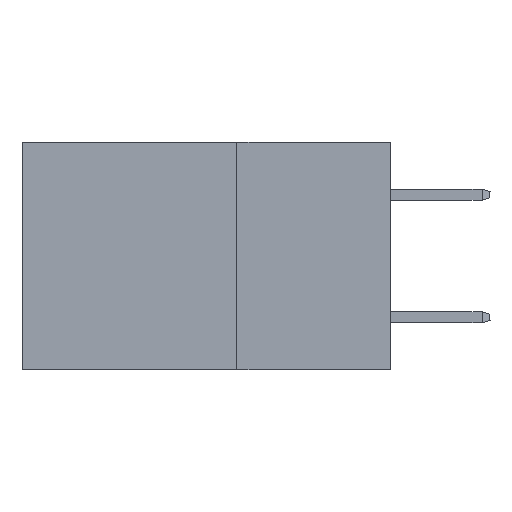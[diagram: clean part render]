
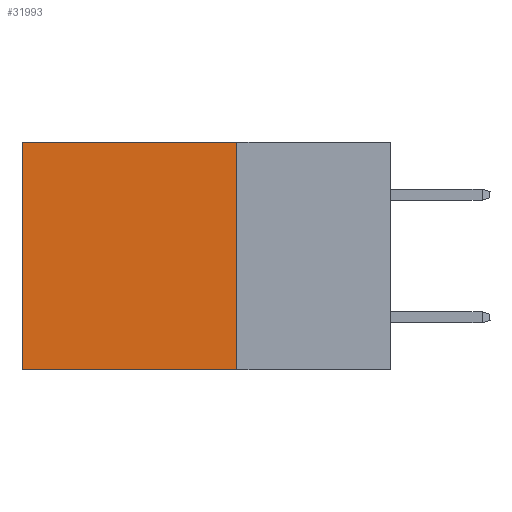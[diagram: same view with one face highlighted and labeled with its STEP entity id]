
A CAD part, left-side view. The second image highlights one B-rep face of the part: STEP entity #31993.
In plain terms, the highlighted planar face has unit normal (-1, 0, 0).
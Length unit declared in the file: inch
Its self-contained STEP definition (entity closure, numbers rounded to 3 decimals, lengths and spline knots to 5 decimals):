
#470 = VECTOR ( 'NONE', #37193, 39.37008 ) ;
#1246 = VECTOR ( 'NONE', #6303, 39.37008 ) ;
#2619 = AXIS2_PLACEMENT_3D ( 'NONE', #25971, #29019, #23151 ) ;
#3380 = VERTEX_POINT ( 'NONE', #5142 ) ;
#3623 = LINE ( 'NONE', #7963, #470 ) ;
#5142 = CARTESIAN_POINT ( 'NONE',  ( 0.2875, 0.25, 0. ) ) ;
#5642 = ORIENTED_EDGE ( 'NONE', *, *, #17626, .F. ) ;
#5778 = VECTOR ( 'NONE', #6934, 39.37008 ) ;
#5882 = CARTESIAN_POINT ( 'NONE',  ( 0.2875, 0.25, -0.37 ) ) ;
#6303 = DIRECTION ( 'NONE',  ( 0., 0., -1. ) ) ;
#6636 = ORIENTED_EDGE ( 'NONE', *, *, #25671, .T. ) ;
#6934 = DIRECTION ( 'NONE',  ( 0., 0., -1. ) ) ;
#7260 = VERTEX_POINT ( 'NONE', #5882 ) ;
#7963 = CARTESIAN_POINT ( 'NONE',  ( 0.2875, 0.25, 0. ) ) ;
#8611 = ORIENTED_EDGE ( 'NONE', *, *, #31252, .T. ) ;
#8920 = LINE ( 'NONE', #23599, #1246 ) ;
#10044 = CARTESIAN_POINT ( 'NONE',  ( 0.2875, 0.25, -0.37 ) ) ;
#10802 = VERTEX_POINT ( 'NONE', #28279 ) ;
#12981 = DIRECTION ( 'NONE',  ( 0., 1., 0. ) ) ;
#13115 = FACE_OUTER_BOUND ( 'NONE', #36855, .T. ) ;
#16904 = CARTESIAN_POINT ( 'NONE',  ( 0.2875, 0.6, 0. ) ) ;
#17626 = EDGE_CURVE ( 'NONE', #7260, #10802, #22421, .T. ) ;
#20752 = ORIENTED_EDGE ( 'NONE', *, *, #25717, .F. ) ;
#22421 = LINE ( 'NONE', #10044, #36909 ) ;
#22670 = VERTEX_POINT ( 'NONE', #16904 ) ;
#23040 = PLANE ( 'NONE',  #2619 ) ;
#23151 = DIRECTION ( 'NONE',  ( 0., 0., -1. ) ) ;
#23599 = CARTESIAN_POINT ( 'NONE',  ( 0.2875, 0.6, 0. ) ) ;
#25671 = EDGE_CURVE ( 'NONE', #22670, #10802, #8920, .T. ) ;
#25717 = EDGE_CURVE ( 'NONE', #3380, #7260, #29814, .T. ) ;
#25971 = CARTESIAN_POINT ( 'NONE',  ( 0.2875, 0.25, 0. ) ) ;
#28279 = CARTESIAN_POINT ( 'NONE',  ( 0.2875, 0.6, -0.37 ) ) ;
#29019 = DIRECTION ( 'NONE',  ( 1., 0., 0. ) ) ;
#29814 = LINE ( 'NONE', #30002, #5778 ) ;
#30002 = CARTESIAN_POINT ( 'NONE',  ( 0.2875, 0.25, 0. ) ) ;
#31252 = EDGE_CURVE ( 'NONE', #3380, #22670, #3623, .T. ) ;
#31993 = ADVANCED_FACE ( 'NONE', ( #13115 ), #23040, .F. ) ;
#36855 = EDGE_LOOP ( 'NONE', ( #6636, #5642, #20752, #8611 ) ) ;
#36909 = VECTOR ( 'NONE', #12981, 39.37008 ) ;
#37193 = DIRECTION ( 'NONE',  ( 0., 1., 0. ) ) ;
